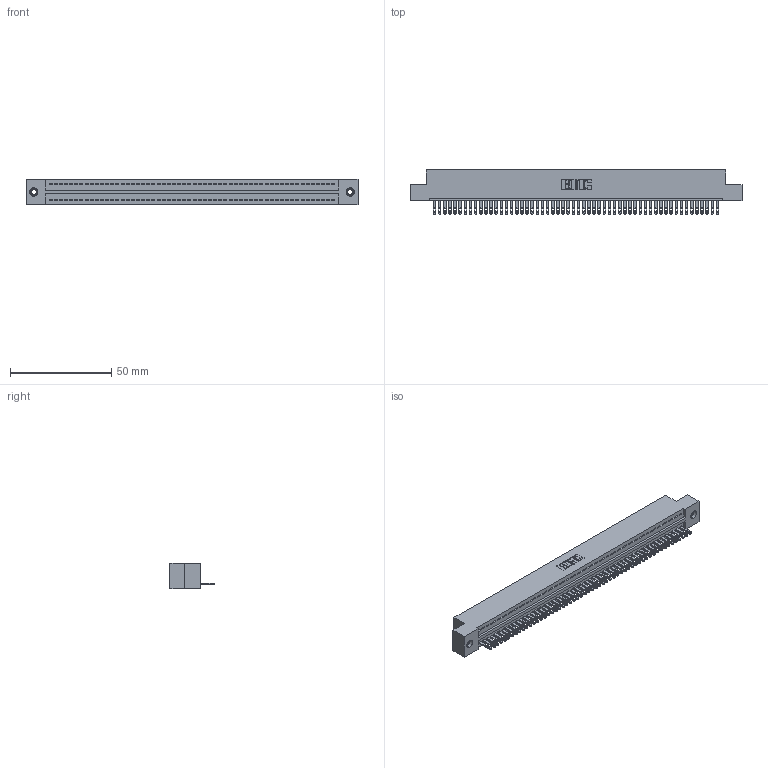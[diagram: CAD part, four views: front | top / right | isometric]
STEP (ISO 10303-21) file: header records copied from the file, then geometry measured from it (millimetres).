
FILE_DESCRIPTION (( 'STEP AP203' ), '1' );
FILE_NAME ('325-056-500-107.STEP', '2020-02-25T01:17:54', ( '' ), ( '' ), 'SwSTEP 2.0', 'SolidWorks 2016', '' );
FILE_SCHEMA (( 'CONFIG_CONTROL_DESIGN' ));
Length unit declared in the file: inch
Products named in the file (4): 325-292-001_325-293-100; 325-056-500-107; 325 Part_TI; 345-250-001_345-250-005-103
Assembly tree (59 placements, depth 2):
  325-056-500-107
    325 Part_TI
    325-292-001_325-293-100  x56
    345-250-001_345-250-005-103  x2
Bounding box: 163.96 x 21.84 x 12.45 mm (x, y, z)
Volume: 20945.7 mm3; surface area: 23279 mm2
Topology: 59 solids, 59 shells, 3198 faces, 9855 edges, 6562 vertices
Faces by surface type: plane 2118, cylinder 1064, cone 12, torus 4
Entity records: 33540 total; most frequent: CARTESIAN_POINT 5765, ORIENTED_EDGE 5750, DIRECTION 4869, EDGE_CURVE 2875, LINE 2723, VECTOR 2723, VERTEX_POINT 1912, AXIS2_PLACEMENT_3D 1073
